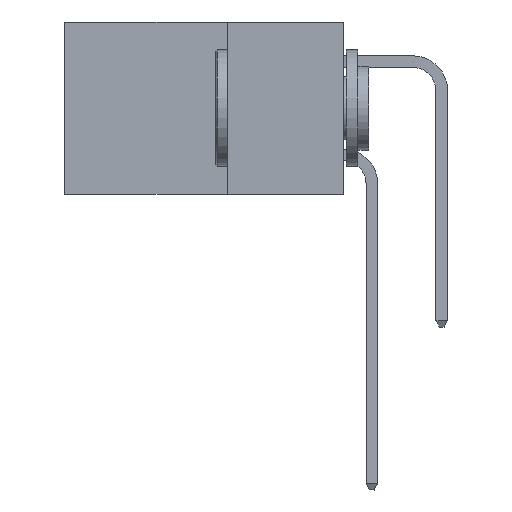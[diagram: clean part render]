
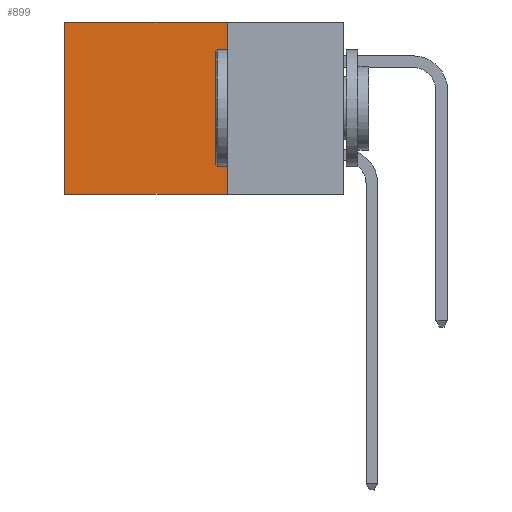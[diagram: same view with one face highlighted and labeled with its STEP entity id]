
A CAD part, left-side view. The second image highlights one B-rep face of the part: STEP entity #899.
In plain terms, the highlighted planar face has unit normal (-1, 0, 0).
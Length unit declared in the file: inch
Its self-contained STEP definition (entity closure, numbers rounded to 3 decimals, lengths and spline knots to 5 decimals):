
#887 = VECTOR ( 'NONE', #5622, 39.37008 ) ;
#899 = ADVANCED_FACE ( 'NONE', ( #5656 ), #15903, .F. ) ;
#2568 = ORIENTED_EDGE ( 'NONE', *, *, #2716, .F. ) ;
#2575 = CARTESIAN_POINT ( 'NONE',  ( 0.298, 0.25, 0. ) ) ;
#2716 = EDGE_CURVE ( 'NONE', #11583, #18395, #8753, .T. ) ;
#3071 = LINE ( 'NONE', #2575, #22337 ) ;
#3292 = ORIENTED_EDGE ( 'NONE', *, *, #4872, .T. ) ;
#3835 = VECTOR ( 'NONE', #6397, 39.37008 ) ;
#4872 = EDGE_CURVE ( 'NONE', #16063, #18395, #18703, .T. ) ;
#5132 = VERTEX_POINT ( 'NONE', #7124 ) ;
#5622 = DIRECTION ( 'NONE',  ( 0., 0., -1. ) ) ;
#5656 = FACE_OUTER_BOUND ( 'NONE', #20689, .T. ) ;
#6397 = DIRECTION ( 'NONE',  ( 0., 1., 0. ) ) ;
#6786 = CARTESIAN_POINT ( 'NONE',  ( 0.298, 0.6, 0. ) ) ;
#7124 = CARTESIAN_POINT ( 'NONE',  ( 0.298, 0.25, 0. ) ) ;
#7390 = EDGE_CURVE ( 'NONE', #5132, #16063, #3071, .T. ) ;
#7975 = DIRECTION ( 'NONE',  ( 0., 0., -1. ) ) ;
#8050 = DIRECTION ( 'NONE',  ( 1., 0., 0. ) ) ;
#8069 = VECTOR ( 'NONE', #13982, 39.37008 ) ;
#8753 = LINE ( 'NONE', #21650, #3835 ) ;
#10485 = ORIENTED_EDGE ( 'NONE', *, *, #13701, .F. ) ;
#10721 = LINE ( 'NONE', #20652, #887 ) ;
#10728 = CARTESIAN_POINT ( 'NONE',  ( 0.298, 0.6, -0.37 ) ) ;
#11043 = DIRECTION ( 'NONE',  ( 0., 1., 0. ) ) ;
#11583 = VERTEX_POINT ( 'NONE', #21300 ) ;
#13701 = EDGE_CURVE ( 'NONE', #5132, #11583, #10721, .T. ) ;
#13982 = DIRECTION ( 'NONE',  ( 0., 0., -1. ) ) ;
#15903 = PLANE ( 'NONE',  #22980 ) ;
#16063 = VERTEX_POINT ( 'NONE', #6786 ) ;
#17573 = CARTESIAN_POINT ( 'NONE',  ( 0.298, 0.25, 0. ) ) ;
#18395 = VERTEX_POINT ( 'NONE', #10728 ) ;
#18703 = LINE ( 'NONE', #20661, #8069 ) ;
#20652 = CARTESIAN_POINT ( 'NONE',  ( 0.298, 0.25, 0. ) ) ;
#20661 = CARTESIAN_POINT ( 'NONE',  ( 0.298, 0.6, 0. ) ) ;
#20689 = EDGE_LOOP ( 'NONE', ( #3292, #2568, #10485, #22432 ) ) ;
#21300 = CARTESIAN_POINT ( 'NONE',  ( 0.298, 0.25, -0.37 ) ) ;
#21650 = CARTESIAN_POINT ( 'NONE',  ( 0.298, 0.25, -0.37 ) ) ;
#22337 = VECTOR ( 'NONE', #11043, 39.37008 ) ;
#22432 = ORIENTED_EDGE ( 'NONE', *, *, #7390, .T. ) ;
#22980 = AXIS2_PLACEMENT_3D ( 'NONE', #17573, #8050, #7975 ) ;
